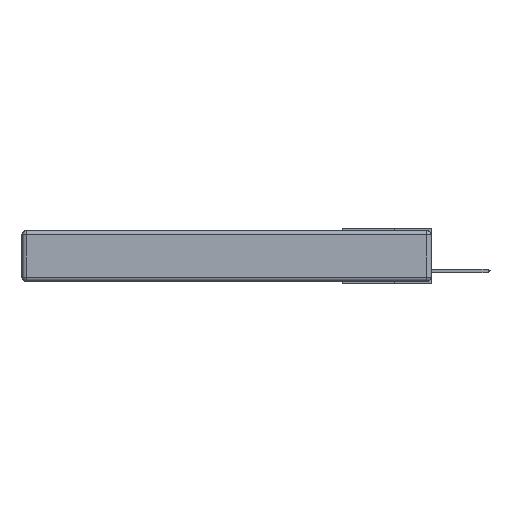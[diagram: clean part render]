
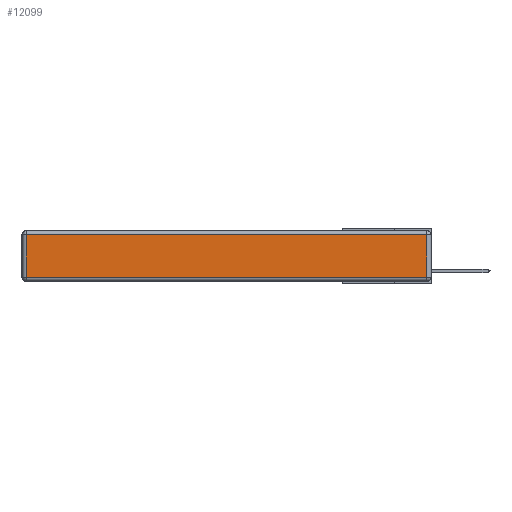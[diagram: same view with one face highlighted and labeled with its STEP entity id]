
A CAD part, left-side view. The second image highlights one B-rep face of the part: STEP entity #12099.
In plain terms, the highlighted planar face has unit normal (-1, 0, 0).
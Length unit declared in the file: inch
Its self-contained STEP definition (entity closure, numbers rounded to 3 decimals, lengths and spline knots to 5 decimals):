
#1292 = CARTESIAN_POINT ( 'NONE',  ( 0., 2.72, -0.343 ) ) ;
#1676 = EDGE_CURVE ( 'NONE', #5896, #19392, #17962, .T. ) ;
#2366 = LINE ( 'NONE', #2397, #18909 ) ;
#2397 = CARTESIAN_POINT ( 'NONE',  ( 0., 2.75, -0.03 ) ) ;
#2545 = VERTEX_POINT ( 'NONE', #10505 ) ;
#2665 = VECTOR ( 'NONE', #15096, 39.37008 ) ;
#2723 = CARTESIAN_POINT ( 'NONE',  ( 0., 0., -0.343 ) ) ;
#4382 = ORIENTED_EDGE ( 'NONE', *, *, #14967, .T. ) ;
#4554 = PLANE ( 'NONE',  #9117 ) ;
#4628 = CARTESIAN_POINT ( 'NONE',  ( 0., 2.72, -0.03 ) ) ;
#5574 = VECTOR ( 'NONE', #7641, 39.37008 ) ;
#5578 = FACE_OUTER_BOUND ( 'NONE', #17760, .T. ) ;
#5896 = VERTEX_POINT ( 'NONE', #4628 ) ;
#6377 = VERTEX_POINT ( 'NONE', #12352 ) ;
#7641 = DIRECTION ( 'NONE',  ( 0., 0., 1. ) ) ;
#8325 = DIRECTION ( 'NONE',  ( -1., 0., 0. ) ) ;
#8422 = ORIENTED_EDGE ( 'NONE', *, *, #1676, .T. ) ;
#9117 = AXIS2_PLACEMENT_3D ( 'NONE', #2723, #8325, #11331 ) ;
#10505 = CARTESIAN_POINT ( 'NONE',  ( 0., 0.03, -0.313 ) ) ;
#10909 = VECTOR ( 'NONE', #19398, 39.37008 ) ;
#11331 = DIRECTION ( 'NONE',  ( 0., 0., 1. ) ) ;
#11435 = LINE ( 'NONE', #19336, #10909 ) ;
#12099 = ADVANCED_FACE ( 'NONE', ( #5578 ), #4554, .T. ) ;
#12352 = CARTESIAN_POINT ( 'NONE',  ( 0., 0.03, -0.03 ) ) ;
#13324 = ORIENTED_EDGE ( 'NONE', *, *, #15805, .T. ) ;
#13432 = DIRECTION ( 'NONE',  ( 0., 1., 0. ) ) ;
#14918 = EDGE_CURVE ( 'NONE', #6377, #5896, #2366, .T. ) ;
#14967 = EDGE_CURVE ( 'NONE', #2545, #6377, #18635, .T. ) ;
#15096 = DIRECTION ( 'NONE',  ( 0., 0., -1. ) ) ;
#15805 = EDGE_CURVE ( 'NONE', #19392, #2545, #11435, .T. ) ;
#17096 = CARTESIAN_POINT ( 'NONE',  ( 0., 0.03, -0.343 ) ) ;
#17760 = EDGE_LOOP ( 'NONE', ( #13324, #4382, #19757, #8422 ) ) ;
#17851 = CARTESIAN_POINT ( 'NONE',  ( 0., 2.72, -0.313 ) ) ;
#17962 = LINE ( 'NONE', #1292, #2665 ) ;
#18635 = LINE ( 'NONE', #17096, #5574 ) ;
#18909 = VECTOR ( 'NONE', #13432, 39.37008 ) ;
#19336 = CARTESIAN_POINT ( 'NONE',  ( 0., 0., -0.313 ) ) ;
#19392 = VERTEX_POINT ( 'NONE', #17851 ) ;
#19398 = DIRECTION ( 'NONE',  ( 0., -1., 0. ) ) ;
#19757 = ORIENTED_EDGE ( 'NONE', *, *, #14918, .T. ) ;
